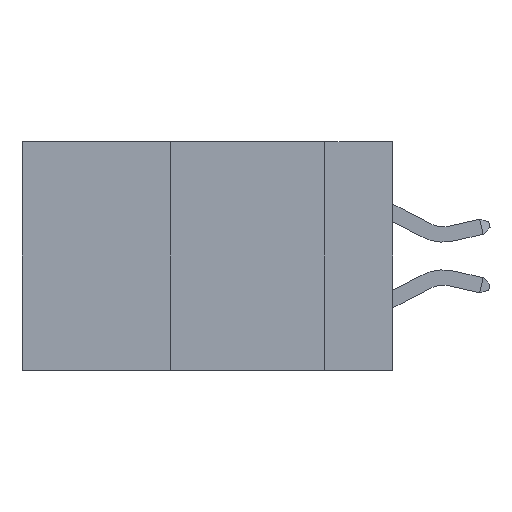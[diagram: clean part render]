
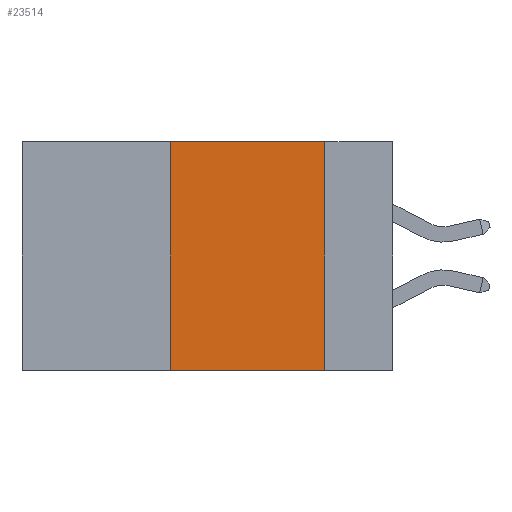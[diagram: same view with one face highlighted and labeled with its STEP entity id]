
A CAD part, left-side view. The second image highlights one B-rep face of the part: STEP entity #23514.
In plain terms, the highlighted planar face has unit normal (-1, 0, 0).
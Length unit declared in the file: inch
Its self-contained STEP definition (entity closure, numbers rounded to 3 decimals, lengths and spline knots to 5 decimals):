
#49 = ORIENTED_EDGE ( 'NONE', *, *, #16520, .T. ) ;
#454 = FACE_OUTER_BOUND ( 'NONE', #7426, .T. ) ;
#1413 = VERTEX_POINT ( 'NONE', #14141 ) ;
#1549 = LINE ( 'NONE', #4597, #20661 ) ;
#1625 = CARTESIAN_POINT ( 'NONE',  ( 0., 0.11, 0. ) ) ;
#2265 = CARTESIAN_POINT ( 'NONE',  ( 0., 0.36, -0.37 ) ) ;
#2756 = AXIS2_PLACEMENT_3D ( 'NONE', #11119, #20143, #3894 ) ;
#2770 = CARTESIAN_POINT ( 'NONE',  ( 0., 0.11, -0.37 ) ) ;
#3375 = CARTESIAN_POINT ( 'NONE',  ( 0., 0.6, 0. ) ) ;
#3894 = DIRECTION ( 'NONE',  ( 0., 0., -1. ) ) ;
#4597 = CARTESIAN_POINT ( 'NONE',  ( 0., 0.36, 0. ) ) ;
#5398 = DIRECTION ( 'NONE',  ( 0., 0., -1. ) ) ;
#7059 = EDGE_CURVE ( 'NONE', #19606, #1413, #1549, .T. ) ;
#7426 = EDGE_LOOP ( 'NONE', ( #8922, #15913, #19686, #49 ) ) ;
#7618 = EDGE_CURVE ( 'NONE', #1413, #18016, #22073, .T. ) ;
#7622 = PLANE ( 'NONE',  #2756 ) ;
#8138 = LINE ( 'NONE', #1625, #21558 ) ;
#8922 = ORIENTED_EDGE ( 'NONE', *, *, #14493, .F. ) ;
#9287 = DIRECTION ( 'NONE',  ( 0., 0., 1. ) ) ;
#11119 = CARTESIAN_POINT ( 'NONE',  ( 0., 0.6, 0. ) ) ;
#12084 = DIRECTION ( 'NONE',  ( 0., -1., 0. ) ) ;
#13034 = CARTESIAN_POINT ( 'NONE',  ( 0., 0.11, 0. ) ) ;
#13566 = VECTOR ( 'NONE', #12084, 39.37008 ) ;
#14141 = CARTESIAN_POINT ( 'NONE',  ( 0., 0.36, 0. ) ) ;
#14493 = EDGE_CURVE ( 'NONE', #18016, #15657, #8138, .T. ) ;
#14759 = DIRECTION ( 'NONE',  ( 0., -1., 0. ) ) ;
#15657 = VERTEX_POINT ( 'NONE', #2770 ) ;
#15913 = ORIENTED_EDGE ( 'NONE', *, *, #7618, .F. ) ;
#16520 = EDGE_CURVE ( 'NONE', #19606, #15657, #18442, .T. ) ;
#18016 = VERTEX_POINT ( 'NONE', #13034 ) ;
#18442 = LINE ( 'NONE', #21036, #13566 ) ;
#19606 = VERTEX_POINT ( 'NONE', #2265 ) ;
#19686 = ORIENTED_EDGE ( 'NONE', *, *, #7059, .F. ) ;
#20143 = DIRECTION ( 'NONE',  ( 1., 0., 0. ) ) ;
#20661 = VECTOR ( 'NONE', #9287, 39.37008 ) ;
#21036 = CARTESIAN_POINT ( 'NONE',  ( 0., 0.6, -0.37 ) ) ;
#21558 = VECTOR ( 'NONE', #5398, 39.37008 ) ;
#22073 = LINE ( 'NONE', #3375, #23476 ) ;
#23476 = VECTOR ( 'NONE', #14759, 39.37008 ) ;
#23514 = ADVANCED_FACE ( 'NONE', ( #454 ), #7622, .F. ) ;
